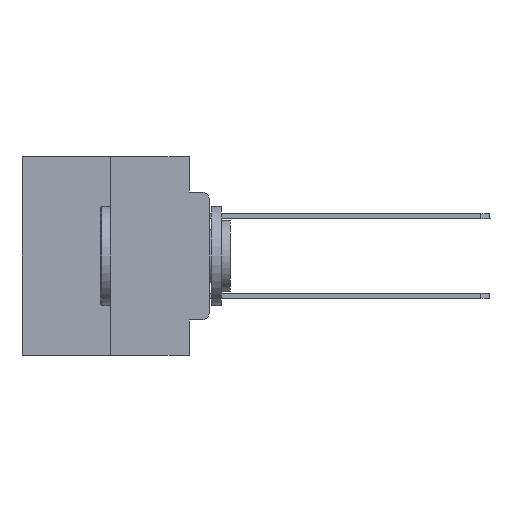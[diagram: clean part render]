
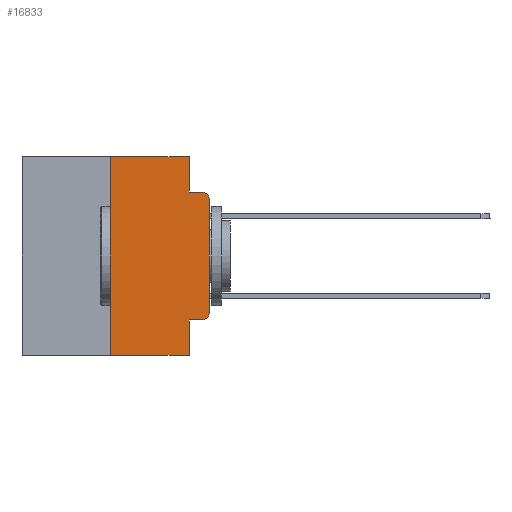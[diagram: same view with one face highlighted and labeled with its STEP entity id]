
A CAD part, left-side view. The second image highlights one B-rep face of the part: STEP entity #16833.
In plain terms, the highlighted planar face has unit normal (-1, 0, 0).
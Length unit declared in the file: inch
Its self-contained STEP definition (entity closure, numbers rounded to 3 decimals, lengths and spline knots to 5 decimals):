
#460 = VECTOR ( 'NONE', #18227, 39.37008 ) ;
#943 = CARTESIAN_POINT ( 'NONE',  ( 0., 0.02, -0.3915 ) ) ;
#990 = ORIENTED_EDGE ( 'NONE', *, *, #9362, .T. ) ;
#1165 = CIRCLE ( 'NONE', #17808, 0.02 ) ;
#1182 = ORIENTED_EDGE ( 'NONE', *, *, #13258, .T. ) ;
#1366 = CARTESIAN_POINT ( 'NONE',  ( 0., 0., -0.3915 ) ) ;
#1448 = ORIENTED_EDGE ( 'NONE', *, *, #22600, .T. ) ;
#1722 = ORIENTED_EDGE ( 'NONE', *, *, #6086, .F. ) ;
#2116 = CARTESIAN_POINT ( 'NONE',  ( 0., 0.051, -0.0885 ) ) ;
#2127 = CARTESIAN_POINT ( 'NONE',  ( 0., 0.02, -0.1085 ) ) ;
#2397 = LINE ( 'NONE', #10823, #24285 ) ;
#2607 = VERTEX_POINT ( 'NONE', #10657 ) ;
#2998 = EDGE_CURVE ( 'NONE', #16422, #18491, #3791, .T. ) ;
#3791 = LINE ( 'NONE', #17107, #29200 ) ;
#3962 = CARTESIAN_POINT ( 'NONE',  ( 0., 0., 0. ) ) ;
#4173 = DIRECTION ( 'NONE',  ( 0., -1., 0. ) ) ;
#4206 = EDGE_LOOP ( 'NONE', ( #1182, #990, #8415, #23329, #1722, #10422, #11859, #11831, #1448, #27898 ) ) ;
#4388 = CARTESIAN_POINT ( 'NONE',  ( 0., 0.051, -0.0885 ) ) ;
#4739 = DIRECTION ( 'NONE',  ( -1., 0., 0. ) ) ;
#5405 = CARTESIAN_POINT ( 'NONE',  ( 0., 0.02, -0.4115 ) ) ;
#5552 = CARTESIAN_POINT ( 'NONE',  ( 0., 0.051, -0.4115 ) ) ;
#5706 = CARTESIAN_POINT ( 'NONE',  ( 0., 0.051, 0. ) ) ;
#6086 = EDGE_CURVE ( 'NONE', #24106, #6845, #7499, .T. ) ;
#6389 = VERTEX_POINT ( 'NONE', #1366 ) ;
#6615 = AXIS2_PLACEMENT_3D ( 'NONE', #2127, #4739, #15789 ) ;
#6833 = CARTESIAN_POINT ( 'NONE',  ( 0., 0., -0.1085 ) ) ;
#6845 = VERTEX_POINT ( 'NONE', #8350 ) ;
#6929 = CARTESIAN_POINT ( 'NONE',  ( 0., 0.25, -0.5 ) ) ;
#7499 = LINE ( 'NONE', #24873, #460 ) ;
#7722 = VECTOR ( 'NONE', #13133, 39.37008 ) ;
#8056 = AXIS2_PLACEMENT_3D ( 'NONE', #15400, #8647, #8738 ) ;
#8067 = FACE_OUTER_BOUND ( 'NONE', #4206, .T. ) ;
#8350 = CARTESIAN_POINT ( 'NONE',  ( 0., 0.051, 0. ) ) ;
#8415 = ORIENTED_EDGE ( 'NONE', *, *, #12079, .F. ) ;
#8647 = DIRECTION ( 'NONE',  ( 1., 0., 0. ) ) ;
#8738 = DIRECTION ( 'NONE',  ( 0., 0., -1. ) ) ;
#9103 = VECTOR ( 'NONE', #23779, 39.37008 ) ;
#9362 = EDGE_CURVE ( 'NONE', #22950, #2607, #11810, .T. ) ;
#9611 = LINE ( 'NONE', #20766, #19867 ) ;
#10422 = ORIENTED_EDGE ( 'NONE', *, *, #11046, .F. ) ;
#10625 = VERTEX_POINT ( 'NONE', #5405 ) ;
#10657 = CARTESIAN_POINT ( 'NONE',  ( 0., 0.02, -0.0885 ) ) ;
#10823 = CARTESIAN_POINT ( 'NONE',  ( 0., 0.051, 0. ) ) ;
#11046 = EDGE_CURVE ( 'NONE', #16422, #24106, #9611, .T. ) ;
#11810 = CIRCLE ( 'NONE', #6615, 0.02 ) ;
#11831 = ORIENTED_EDGE ( 'NONE', *, *, #17175, .F. ) ;
#11859 = ORIENTED_EDGE ( 'NONE', *, *, #2998, .T. ) ;
#11871 = EDGE_CURVE ( 'NONE', #10625, #6389, #1165, .T. ) ;
#12079 = EDGE_CURVE ( 'NONE', #18021, #2607, #21603, .T. ) ;
#12538 = DIRECTION ( 'NONE',  ( 0., 0., -1. ) ) ;
#12662 = CARTESIAN_POINT ( 'NONE',  ( 0., 0.051, -0.4115 ) ) ;
#13133 = DIRECTION ( 'NONE',  ( 0., 0., 1. ) ) ;
#13258 = EDGE_CURVE ( 'NONE', #6389, #22950, #23280, .T. ) ;
#13912 = VECTOR ( 'NONE', #28463, 39.37008 ) ;
#15400 = CARTESIAN_POINT ( 'NONE',  ( 0., 0.473, 0. ) ) ;
#15590 = VECTOR ( 'NONE', #4173, 39.37008 ) ;
#15789 = DIRECTION ( 'NONE',  ( 0., 0., -1. ) ) ;
#15918 = CARTESIAN_POINT ( 'NONE',  ( 0., 0.25, 0. ) ) ;
#16245 = DIRECTION ( 'NONE',  ( 0., 0., 1. ) ) ;
#16422 = VERTEX_POINT ( 'NONE', #6929 ) ;
#16686 = DIRECTION ( 'NONE',  ( -1., 0., 0. ) ) ;
#16833 = ADVANCED_FACE ( 'NONE', ( #8067 ), #17659, .F. ) ;
#17107 = CARTESIAN_POINT ( 'NONE',  ( 0., 0.473, -0.5 ) ) ;
#17175 = EDGE_CURVE ( 'NONE', #28416, #18491, #18673, .T. ) ;
#17659 = PLANE ( 'NONE',  #8056 ) ;
#17791 = LINE ( 'NONE', #12662, #13912 ) ;
#17808 = AXIS2_PLACEMENT_3D ( 'NONE', #943, #16686, #12538 ) ;
#18021 = VERTEX_POINT ( 'NONE', #4388 ) ;
#18227 = DIRECTION ( 'NONE',  ( 0., -1., 0. ) ) ;
#18491 = VERTEX_POINT ( 'NONE', #21637 ) ;
#18673 = LINE ( 'NONE', #5706, #9103 ) ;
#19579 = DIRECTION ( 'NONE',  ( 0., -1., 0. ) ) ;
#19867 = VECTOR ( 'NONE', #16245, 39.37008 ) ;
#20766 = CARTESIAN_POINT ( 'NONE',  ( 0., 0.25, 0. ) ) ;
#21603 = LINE ( 'NONE', #2116, #15590 ) ;
#21637 = CARTESIAN_POINT ( 'NONE',  ( 0., 0.051, -0.5 ) ) ;
#22195 = DIRECTION ( 'NONE',  ( 0., 0., -1. ) ) ;
#22600 = EDGE_CURVE ( 'NONE', #28416, #10625, #17791, .T. ) ;
#22950 = VERTEX_POINT ( 'NONE', #6833 ) ;
#23280 = LINE ( 'NONE', #3962, #7722 ) ;
#23329 = ORIENTED_EDGE ( 'NONE', *, *, #27101, .F. ) ;
#23779 = DIRECTION ( 'NONE',  ( 0., 0., -1. ) ) ;
#24106 = VERTEX_POINT ( 'NONE', #15918 ) ;
#24285 = VECTOR ( 'NONE', #22195, 39.37008 ) ;
#24873 = CARTESIAN_POINT ( 'NONE',  ( 0., 0.473, 0. ) ) ;
#27101 = EDGE_CURVE ( 'NONE', #6845, #18021, #2397, .T. ) ;
#27898 = ORIENTED_EDGE ( 'NONE', *, *, #11871, .T. ) ;
#28416 = VERTEX_POINT ( 'NONE', #5552 ) ;
#28463 = DIRECTION ( 'NONE',  ( 0., -1., 0. ) ) ;
#29200 = VECTOR ( 'NONE', #19579, 39.37008 ) ;
